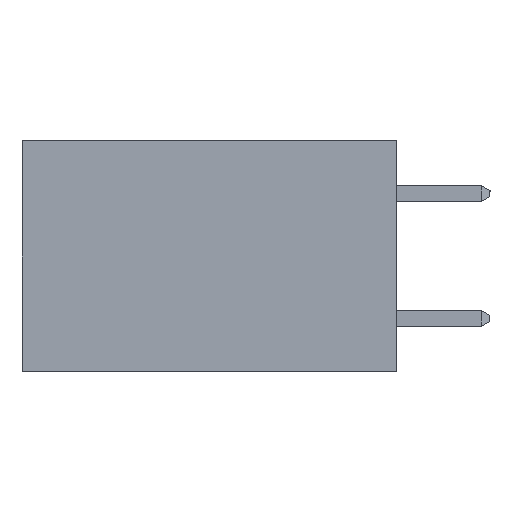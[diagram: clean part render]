
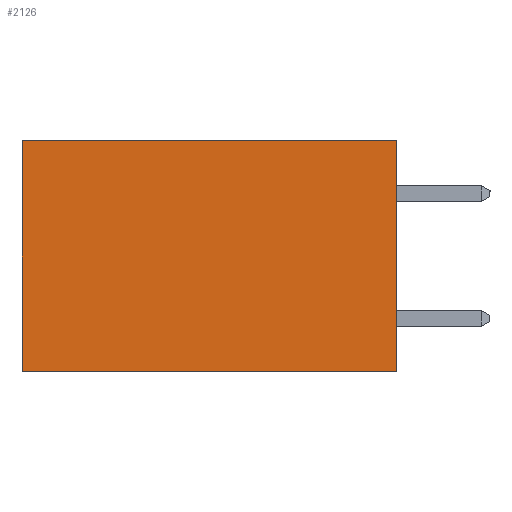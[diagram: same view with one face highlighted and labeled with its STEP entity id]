
A CAD part, left-side view. The second image highlights one B-rep face of the part: STEP entity #2126.
In plain terms, the highlighted planar face has unit normal (-1, 0, 0).
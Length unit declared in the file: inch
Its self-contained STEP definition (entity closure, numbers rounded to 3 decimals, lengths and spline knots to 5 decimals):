
#304 = VERTEX_POINT ( 'NONE', #11008 ) ;
#327 = PLANE ( 'NONE',  #487 ) ;
#487 = AXIS2_PLACEMENT_3D ( 'NONE', #1635, #13790, #3771 ) ;
#562 = VERTEX_POINT ( 'NONE', #7869 ) ;
#1402 = ORIENTED_EDGE ( 'NONE', *, *, #9959, .F. ) ;
#1513 = LINE ( 'NONE', #7159, #9695 ) ;
#1528 = CARTESIAN_POINT ( 'NONE',  ( 0.2615, 0.6, -0.37 ) ) ;
#1635 = CARTESIAN_POINT ( 'NONE',  ( 0.2615, 0., -0.37 ) ) ;
#2126 = ADVANCED_FACE ( 'NONE', ( #11670 ), #327, .F. ) ;
#2301 = LINE ( 'NONE', #13335, #5494 ) ;
#2380 = DIRECTION ( 'NONE',  ( 0., 1., 0. ) ) ;
#2702 = LINE ( 'NONE', #13020, #11828 ) ;
#3218 = LINE ( 'NONE', #13572, #13170 ) ;
#3771 = DIRECTION ( 'NONE',  ( 0., 0., -1. ) ) ;
#5494 = VECTOR ( 'NONE', #5740, 39.37008 ) ;
#5613 = EDGE_LOOP ( 'NONE', ( #11575, #8208, #1402, #8399 ) ) ;
#5689 = CARTESIAN_POINT ( 'NONE',  ( 0.2615, 0.6, 0. ) ) ;
#5740 = DIRECTION ( 'NONE',  ( 0., 1., 0. ) ) ;
#6356 = VERTEX_POINT ( 'NONE', #5689 ) ;
#7159 = CARTESIAN_POINT ( 'NONE',  ( 0.2615, 0., -0.37 ) ) ;
#7457 = DIRECTION ( 'NONE',  ( 0., 0., -1. ) ) ;
#7869 = CARTESIAN_POINT ( 'NONE',  ( 0.2615, 0., -0.37 ) ) ;
#8118 = EDGE_CURVE ( 'NONE', #304, #6356, #3218, .T. ) ;
#8208 = ORIENTED_EDGE ( 'NONE', *, *, #12139, .F. ) ;
#8399 = ORIENTED_EDGE ( 'NONE', *, *, #8118, .T. ) ;
#9487 = VERTEX_POINT ( 'NONE', #1528 ) ;
#9695 = VECTOR ( 'NONE', #10663, 39.37008 ) ;
#9959 = EDGE_CURVE ( 'NONE', #304, #562, #1513, .T. ) ;
#10663 = DIRECTION ( 'NONE',  ( 0., 0., -1. ) ) ;
#10862 = EDGE_CURVE ( 'NONE', #6356, #9487, #2702, .T. ) ;
#11008 = CARTESIAN_POINT ( 'NONE',  ( 0.2615, 0., 0. ) ) ;
#11575 = ORIENTED_EDGE ( 'NONE', *, *, #10862, .T. ) ;
#11670 = FACE_OUTER_BOUND ( 'NONE', #5613, .T. ) ;
#11828 = VECTOR ( 'NONE', #7457, 39.37008 ) ;
#12139 = EDGE_CURVE ( 'NONE', #562, #9487, #2301, .T. ) ;
#13020 = CARTESIAN_POINT ( 'NONE',  ( 0.2615, 0.6, -0.37 ) ) ;
#13170 = VECTOR ( 'NONE', #2380, 39.37008 ) ;
#13335 = CARTESIAN_POINT ( 'NONE',  ( 0.2615, 0., -0.37 ) ) ;
#13572 = CARTESIAN_POINT ( 'NONE',  ( 0.2615, 0., 0. ) ) ;
#13790 = DIRECTION ( 'NONE',  ( 1., 0., 0. ) ) ;
